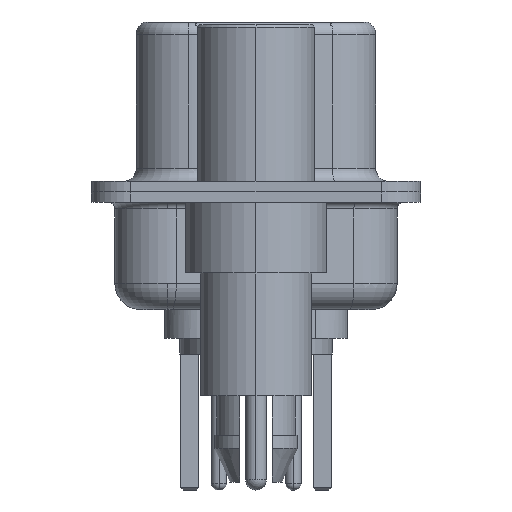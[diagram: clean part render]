
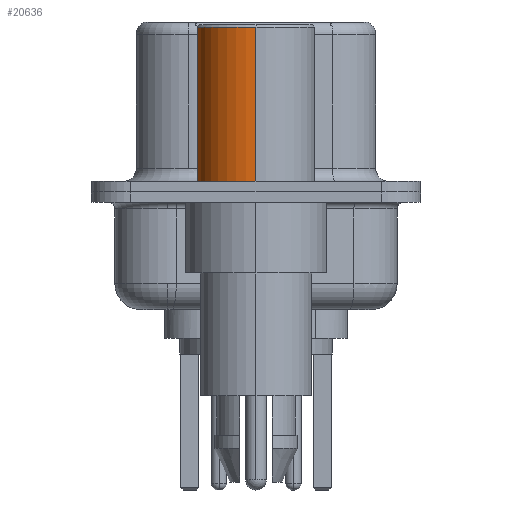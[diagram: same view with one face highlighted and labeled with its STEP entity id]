
A CAD part, left-side view. The second image highlights one B-rep face of the part: STEP entity #20636.
In plain terms, the highlighted cylindrical face has radius 2.25 mm (diameter 4.5 mm), a partial arc.
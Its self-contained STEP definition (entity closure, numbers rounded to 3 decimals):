
#283 = VERTEX_POINT ( 'NONE', #10263 ) ;
#397 = AXIS2_PLACEMENT_3D ( 'NONE', #13471, #1175, #15496 ) ;
#851 = ORIENTED_EDGE ( 'NONE', *, *, #22056, .F. ) ;
#1016 = VERTEX_POINT ( 'NONE', #22640 ) ;
#1175 = DIRECTION ( 'NONE',  ( 0., 0., 1. ) ) ;
#1291 = CARTESIAN_POINT ( 'NONE',  ( -2.25, 0., 0.4 ) ) ;
#2066 = CARTESIAN_POINT ( 'NONE',  ( 2.25, 0., 0.581 ) ) ;
#2732 = DIRECTION ( 'NONE',  ( 0., 0., 1. ) ) ;
#4379 = FACE_OUTER_BOUND ( 'NONE', #10347, .T. ) ;
#4744 = CARTESIAN_POINT ( 'NONE',  ( 0., 0., 0.581 ) ) ;
#5153 = VERTEX_POINT ( 'NONE', #9560 ) ;
#5966 = AXIS2_PLACEMENT_3D ( 'NONE', #8937, #23065, #11008 ) ;
#6683 = ORIENTED_EDGE ( 'NONE', *, *, #25366, .T. ) ;
#8937 = CARTESIAN_POINT ( 'NONE',  ( 0., 0., 0.4 ) ) ;
#9052 = VECTOR ( 'NONE', #22372, 1000. ) ;
#9560 = CARTESIAN_POINT ( 'NONE',  ( -2.25, 0., 6.3 ) ) ;
#10263 = CARTESIAN_POINT ( 'NONE',  ( 2.25, 0., 0.4 ) ) ;
#10347 = EDGE_LOOP ( 'NONE', ( #6683, #16114, #851, #22761 ) ) ;
#10560 = EDGE_CURVE ( 'NONE', #283, #1016, #14508, .T. ) ;
#11008 = DIRECTION ( 'NONE',  ( 1., 0., 0. ) ) ;
#12584 = AXIS2_PLACEMENT_3D ( 'NONE', #4744, #2732, #16994 ) ;
#13471 = CARTESIAN_POINT ( 'NONE',  ( 0., 0., 6.3 ) ) ;
#14504 = VERTEX_POINT ( 'NONE', #1291 ) ;
#14508 = LINE ( 'NONE', #2066, #9052 ) ;
#14590 = CYLINDRICAL_SURFACE ( 'NONE', #12584, 2.25 ) ;
#15496 = DIRECTION ( 'NONE',  ( 1., 0., 0. ) ) ;
#16114 = ORIENTED_EDGE ( 'NONE', *, *, #22713, .T. ) ;
#16200 = DIRECTION ( 'NONE',  ( 0., 0., 1. ) ) ;
#16631 = CIRCLE ( 'NONE', #5966, 2.25 ) ;
#16994 = DIRECTION ( 'NONE',  ( 1., 0., 0. ) ) ;
#20515 = CIRCLE ( 'NONE', #397, 2.25 ) ;
#20636 = ADVANCED_FACE ( 'NONE', ( #4379 ), #14590, .T. ) ;
#22056 = EDGE_CURVE ( 'NONE', #1016, #5153, #20515, .T. ) ;
#22372 = DIRECTION ( 'NONE',  ( 0., 0., 1. ) ) ;
#22631 = LINE ( 'NONE', #24122, #22646 ) ;
#22640 = CARTESIAN_POINT ( 'NONE',  ( 2.25, 0., 6.3 ) ) ;
#22646 = VECTOR ( 'NONE', #16200, 1000. ) ;
#22713 = EDGE_CURVE ( 'NONE', #14504, #5153, #22631, .T. ) ;
#22761 = ORIENTED_EDGE ( 'NONE', *, *, #10560, .F. ) ;
#23065 = DIRECTION ( 'NONE',  ( 0., 0., 1. ) ) ;
#24122 = CARTESIAN_POINT ( 'NONE',  ( -2.25, 0., 0.581 ) ) ;
#25366 = EDGE_CURVE ( 'NONE', #283, #14504, #16631, .T. ) ;
